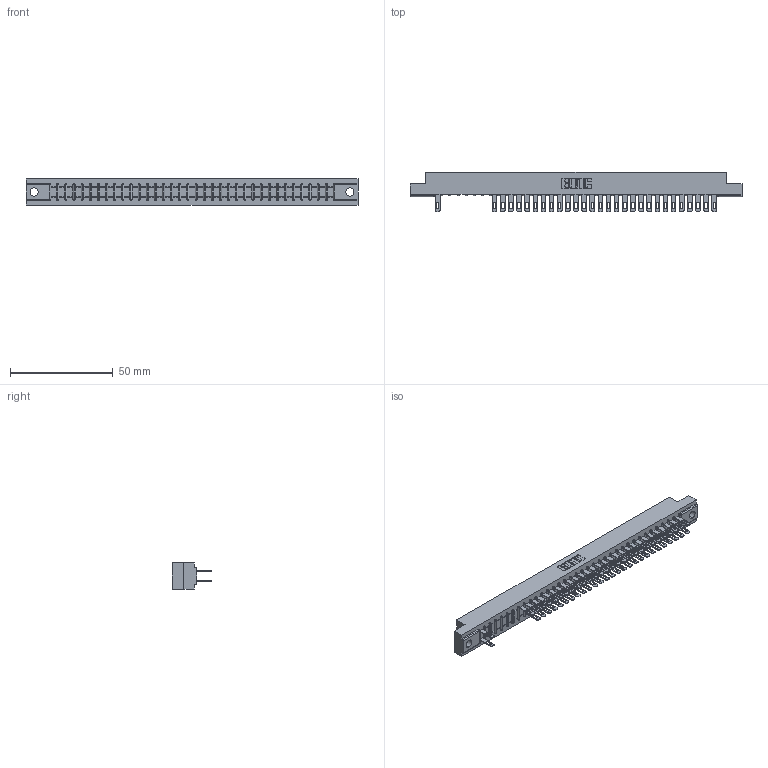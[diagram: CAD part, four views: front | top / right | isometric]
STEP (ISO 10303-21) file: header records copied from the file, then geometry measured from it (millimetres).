
FILE_DESCRIPTION (( 'STEP AP203' ), '1' );
FILE_NAME ('307-070-500-204.STEP', '2018-08-06T12:36:58', ( '' ), ( '' ), 'SwSTEP 2.0', 'SolidWorks 2016', '' );
FILE_SCHEMA (( 'CONFIG_CONTROL_DESIGN' ));
Length unit declared in the file: inch
Products named in the file (3): 307 Part_.156 Dia Mounting Holes; 307-290-001_500; 307-070-500-204
Assembly tree (58 placements, depth 2):
  307-070-500-204
    307 Part_.156 Dia Mounting Holes
    307-290-001_500  x57
Bounding box: 161.7 x 19.18 x 12.7 mm (x, y, z)
Volume: 17033.9 mm3; surface area: 20336 mm2
Topology: 58 solids, 58 shells, 2920 faces, 8185 edges, 5282 vertices
Faces by surface type: plane 1872, cylinder 976, sphere 72
Entity records: 31964 total; most frequent: CARTESIAN_POINT 5288, ORIENTED_EDGE 5250, DIRECTION 5163, EDGE_CURVE 2625, LINE 2017, VECTOR 2017, VERTEX_POINT 1698, AXIS2_PLACEMENT_3D 1573
